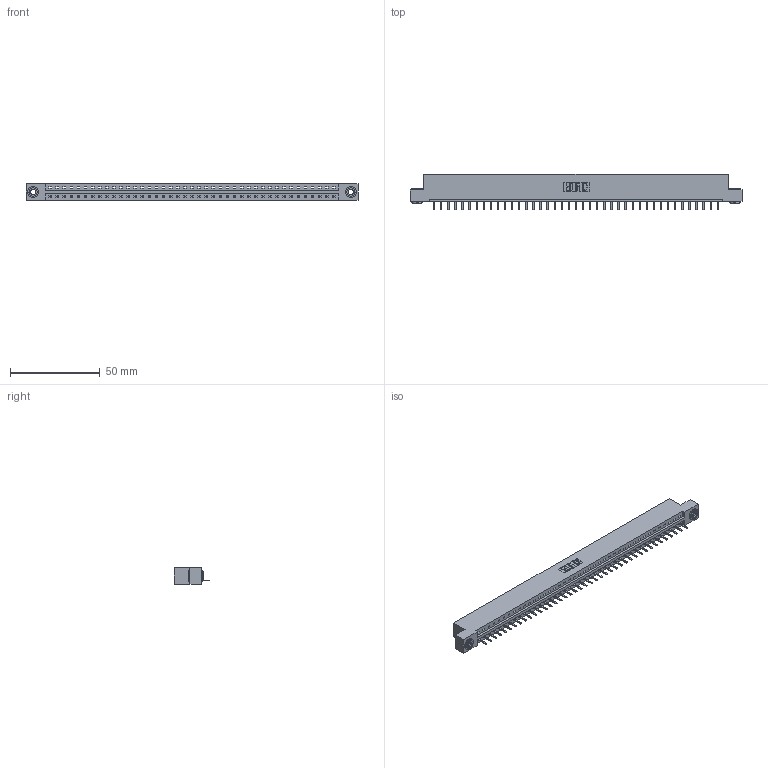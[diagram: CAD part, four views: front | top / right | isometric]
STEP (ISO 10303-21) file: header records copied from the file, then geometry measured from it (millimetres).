
FILE_DESCRIPTION (( 'STEP AP203' ), '1' );
FILE_NAME ('387-041-520-103.STEP', '2019-10-04T19:17:50', ( '' ), ( '' ), 'SwSTEP 2.0', 'SolidWorks 2016', '' );
FILE_SCHEMA (( 'CONFIG_CONTROL_DESIGN' ));
Length unit declared in the file: inch
Products named in the file (4): 387-041-520-103; 337 Part_Flush Mounting Lugs - 0.156 Dia-TH; 345-292-001_345-293-120; 345-250-002_345-250-002-102
Assembly tree (44 placements, depth 2):
  387-041-520-103
    337 Part_Flush Mounting Lugs - 0.156 Dia-TH
    345-292-001_345-293-120  x41
    345-250-002_345-250-002-102  x2
Bounding box: 185.47 x 20.02 x 9.4 mm (x, y, z)
Volume: 19165.5 mm3; surface area: 19607.4 mm2
Topology: 44 solids, 44 shells, 2858 faces, 8423 edges, 5502 vertices
Faces by surface type: plane 2048, cylinder 802, cone 8
Entity records: 31370 total; most frequent: CARTESIAN_POINT 5452, ORIENTED_EDGE 5410, DIRECTION 4613, EDGE_CURVE 2705, LINE 2549, VECTOR 2549, VERTEX_POINT 1798, AXIS2_PLACEMENT_3D 1032
